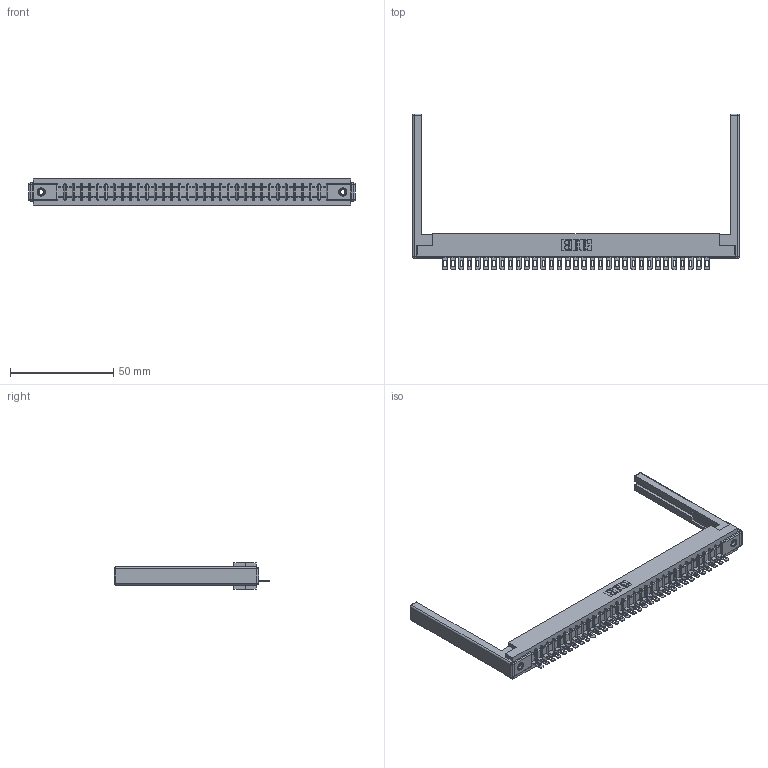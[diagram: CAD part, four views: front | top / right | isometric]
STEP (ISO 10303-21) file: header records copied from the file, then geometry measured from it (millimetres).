
FILE_DESCRIPTION (( 'STEP AP203' ), '1' );
FILE_NAME ('357-033-501-168.STEP', '2019-09-17T04:41:33', ( '' ), ( '' ), 'SwSTEP 2.0', 'SolidWorks 2016', '' );
FILE_SCHEMA (( 'CONFIG_CONTROL_DESIGN' ));
Length unit declared in the file: inch
Products named in the file (5): 357-033-501-168; 307-220-068; 307-290-002_501; 307 Part_.156 Dia Mounting Holes; 345-250-001_345-250-001-102
Assembly tree (38 placements, depth 2):
  357-033-501-168
    307 Part_.156 Dia Mounting Holes
    307-290-002_501  x33
    307-220-068  x2
    345-250-001_345-250-001-102  x2
Bounding box: 158.19 x 75.39 x 12.7 mm (x, y, z)
Volume: 21267.7 mm3; surface area: 25223.9 mm2
Topology: 38 solids, 38 shells, 2814 faces, 8567 edges, 5598 vertices
Faces by surface type: plane 1610, cylinder 1112, sphere 76, cone 12, torus 4
Entity records: 32953 total; most frequent: CARTESIAN_POINT 5521, ORIENTED_EDGE 5500, DIRECTION 5390, EDGE_CURVE 2750, VECTOR 2096, LINE 2096, VERTEX_POINT 1778, AXIS2_PLACEMENT_3D 1647
